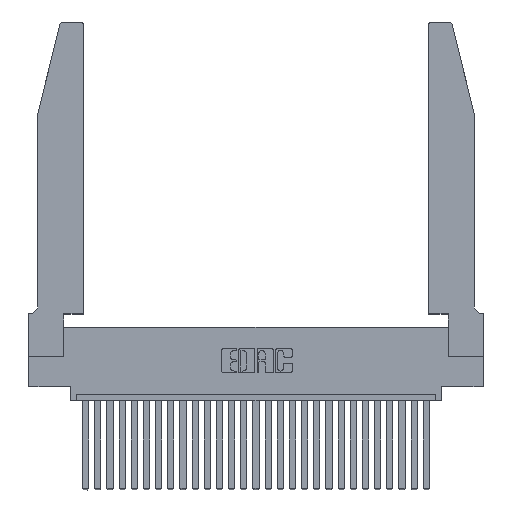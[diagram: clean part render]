
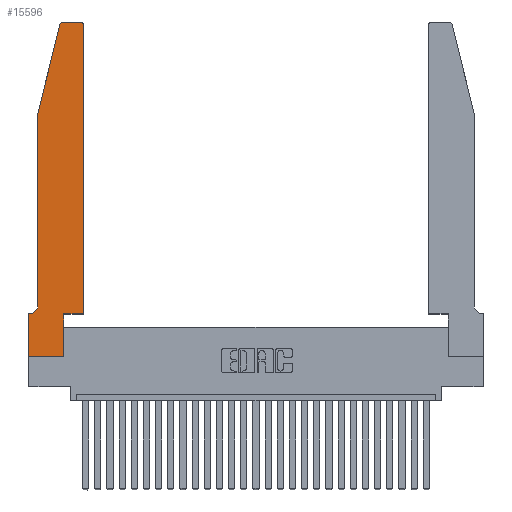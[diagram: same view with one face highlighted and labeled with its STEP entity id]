
A CAD part, top view. The second image highlights one B-rep face of the part: STEP entity #15596.
In plain terms, the highlighted planar face has unit normal (0, 0, 1).
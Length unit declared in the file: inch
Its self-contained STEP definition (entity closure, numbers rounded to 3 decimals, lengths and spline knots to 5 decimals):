
#415 = DIRECTION ( 'NONE',  ( 1., 0., 0. ) ) ;
#1036 = CARTESIAN_POINT ( 'NONE',  ( 0., 0.35, 0.37 ) ) ;
#1130 = LINE ( 'NONE', #27036, #25016 ) ;
#1183 = DIRECTION ( 'NONE',  ( 0., -1., 0. ) ) ;
#1680 = AXIS2_PLACEMENT_3D ( 'NONE', #26564, #13451, #415 ) ;
#1920 = CARTESIAN_POINT ( 'NONE',  ( 0.4505, 0.35, 0.37 ) ) ;
#2234 = VERTEX_POINT ( 'NONE', #7992 ) ;
#2276 = EDGE_CURVE ( 'NONE', #23828, #10349, #15919, .T. ) ;
#2674 = CARTESIAN_POINT ( 'NONE',  ( 0.2865, 0.35, 0.37 ) ) ;
#3351 = CARTESIAN_POINT ( 'NONE',  ( 0.25487, 2.72718, 0.37 ) ) ;
#3857 = VERTEX_POINT ( 'NONE', #1036 ) ;
#3939 = CARTESIAN_POINT ( 'NONE',  ( 0.0755, 2., 0.37 ) ) ;
#4327 = VERTEX_POINT ( 'NONE', #22455 ) ;
#4660 = AXIS2_PLACEMENT_3D ( 'NONE', #6257, #19275, #23594 ) ;
#5125 = CARTESIAN_POINT ( 'NONE',  ( 0.2605, 2.75, 0.37 ) ) ;
#5179 = CARTESIAN_POINT ( 'NONE',  ( 0.2865, 0.35, 0.37 ) ) ;
#5183 = CARTESIAN_POINT ( 'NONE',  ( 0.4505, 2.72, 0.37 ) ) ;
#5343 = VECTOR ( 'NONE', #1183, 39.37008 ) ;
#5871 = ORIENTED_EDGE ( 'NONE', *, *, #2276, .T. ) ;
#6257 = CARTESIAN_POINT ( 'NONE',  ( 0.0055, 0.42, 0.37 ) ) ;
#6505 = CARTESIAN_POINT ( 'NONE',  ( 0.4205, 2.72, 0.37 ) ) ;
#6603 = EDGE_LOOP ( 'NONE', ( #27213, #22534, #7168, #23270, #9719, #13667, #22510, #10000, #21009, #5871, #13877, #24742 ) ) ;
#7168 = ORIENTED_EDGE ( 'NONE', *, *, #11654, .T. ) ;
#7388 = LINE ( 'NONE', #27141, #5343 ) ;
#7731 = DIRECTION ( 'NONE',  ( -0.239, -0.971, 0. ) ) ;
#7992 = CARTESIAN_POINT ( 'NONE',  ( 0., 0., 0.37 ) ) ;
#8528 = VECTOR ( 'NONE', #26946, 39.37008 ) ;
#8648 = EDGE_CURVE ( 'NONE', #10349, #11797, #23971, .T. ) ;
#8759 = CARTESIAN_POINT ( 'NONE',  ( 0.4505, 0.35, 0.37 ) ) ;
#8798 = DIRECTION ( 'NONE',  ( 1., 0., 0. ) ) ;
#8976 = AXIS2_PLACEMENT_3D ( 'NONE', #15329, #25448, #24023 ) ;
#9004 = CARTESIAN_POINT ( 'NONE',  ( 0.0755, 0.42, 0.37 ) ) ;
#9065 = CIRCLE ( 'NONE', #22004, 0.03 ) ;
#9530 = LINE ( 'NONE', #5125, #8528 ) ;
#9719 = ORIENTED_EDGE ( 'NONE', *, *, #20926, .T. ) ;
#9787 = CARTESIAN_POINT ( 'NONE',  ( 0., 0., 0.37 ) ) ;
#10000 = ORIENTED_EDGE ( 'NONE', *, *, #12123, .T. ) ;
#10050 = VECTOR ( 'NONE', #7731, 39.37008 ) ;
#10331 = EDGE_CURVE ( 'NONE', #12961, #4327, #9530, .T. ) ;
#10349 = VERTEX_POINT ( 'NONE', #26844 ) ;
#10372 = DIRECTION ( 'NONE',  ( 1., 0., 0. ) ) ;
#11444 = EDGE_CURVE ( 'NONE', #12896, #23828, #17238, .T. ) ;
#11583 = VERTEX_POINT ( 'NONE', #9004 ) ;
#11654 = EDGE_CURVE ( 'NONE', #22924, #15992, #23799, .T. ) ;
#11797 = VERTEX_POINT ( 'NONE', #5183 ) ;
#12123 = EDGE_CURVE ( 'NONE', #2234, #12896, #21019, .T. ) ;
#12896 = VERTEX_POINT ( 'NONE', #19856 ) ;
#12961 = VERTEX_POINT ( 'NONE', #27208 ) ;
#13053 = EDGE_CURVE ( 'NONE', #4327, #22924, #23366, .T. ) ;
#13451 = DIRECTION ( 'NONE',  ( 0., 0., 1. ) ) ;
#13667 = ORIENTED_EDGE ( 'NONE', *, *, #21769, .T. ) ;
#13877 = ORIENTED_EDGE ( 'NONE', *, *, #8648, .T. ) ;
#14524 = EDGE_CURVE ( 'NONE', #15992, #11583, #7388, .T. ) ;
#14674 = CARTESIAN_POINT ( 'NONE',  ( 0.0055, 0.35, 0.37 ) ) ;
#15329 = CARTESIAN_POINT ( 'NONE',  ( 0., 0.35, 0.37 ) ) ;
#15385 = LINE ( 'NONE', #24969, #17817 ) ;
#15596 = ADVANCED_FACE ( 'NONE', ( #27909 ), #17480, .T. ) ;
#15919 = LINE ( 'NONE', #8759, #25504 ) ;
#15992 = VERTEX_POINT ( 'NONE', #3939 ) ;
#17238 = LINE ( 'NONE', #2674, #23065 ) ;
#17480 = PLANE ( 'NONE',  #8976 ) ;
#17491 = DIRECTION ( 'NONE',  ( 0., 0., 1. ) ) ;
#17817 = VECTOR ( 'NONE', #24889, 39.37008 ) ;
#18172 = VERTEX_POINT ( 'NONE', #14674 ) ;
#19275 = DIRECTION ( 'NONE',  ( 0., 0., -1. ) ) ;
#19856 = CARTESIAN_POINT ( 'NONE',  ( 0.2865, 0., 0.37 ) ) ;
#20667 = CARTESIAN_POINT ( 'NONE',  ( 0.0755, 2., 0.37 ) ) ;
#20926 = EDGE_CURVE ( 'NONE', #11583, #18172, #26381, .T. ) ;
#21009 = ORIENTED_EDGE ( 'NONE', *, *, #11444, .T. ) ;
#21019 = LINE ( 'NONE', #9787, #24769 ) ;
#21495 = EDGE_CURVE ( 'NONE', #3857, #2234, #15385, .T. ) ;
#21769 = EDGE_CURVE ( 'NONE', #18172, #3857, #1130, .T. ) ;
#22004 = AXIS2_PLACEMENT_3D ( 'NONE', #6505, #17491, #8798 ) ;
#22455 = CARTESIAN_POINT ( 'NONE',  ( 0.284, 2.75, 0.37 ) ) ;
#22510 = ORIENTED_EDGE ( 'NONE', *, *, #21495, .T. ) ;
#22534 = ORIENTED_EDGE ( 'NONE', *, *, #13053, .T. ) ;
#22924 = VERTEX_POINT ( 'NONE', #3351 ) ;
#23065 = VECTOR ( 'NONE', #24344, 39.37008 ) ;
#23270 = ORIENTED_EDGE ( 'NONE', *, *, #14524, .T. ) ;
#23366 = CIRCLE ( 'NONE', #1680, 0.03 ) ;
#23594 = DIRECTION ( 'NONE',  ( -1., 0., 0. ) ) ;
#23799 = LINE ( 'NONE', #20667, #10050 ) ;
#23828 = VERTEX_POINT ( 'NONE', #5179 ) ;
#23971 = LINE ( 'NONE', #1920, #27395 ) ;
#24023 = DIRECTION ( 'NONE',  ( 1., 0., 0. ) ) ;
#24058 = DIRECTION ( 'NONE',  ( 1., 0., 0. ) ) ;
#24344 = DIRECTION ( 'NONE',  ( 0., 1., 0. ) ) ;
#24742 = ORIENTED_EDGE ( 'NONE', *, *, #27731, .T. ) ;
#24769 = VECTOR ( 'NONE', #10372, 39.37008 ) ;
#24889 = DIRECTION ( 'NONE',  ( 0., -1., 0. ) ) ;
#24919 = DIRECTION ( 'NONE',  ( -1., 0., 0. ) ) ;
#24969 = CARTESIAN_POINT ( 'NONE',  ( 0., 0., 0.37 ) ) ;
#25016 = VECTOR ( 'NONE', #24919, 39.37008 ) ;
#25448 = DIRECTION ( 'NONE',  ( 0., 0., 1. ) ) ;
#25504 = VECTOR ( 'NONE', #24058, 39.37008 ) ;
#26381 = CIRCLE ( 'NONE', #4660, 0.07 ) ;
#26516 = DIRECTION ( 'NONE',  ( 0., 1., 0. ) ) ;
#26564 = CARTESIAN_POINT ( 'NONE',  ( 0.284, 2.72, 0.37 ) ) ;
#26844 = CARTESIAN_POINT ( 'NONE',  ( 0.4505, 0.35, 0.37 ) ) ;
#26946 = DIRECTION ( 'NONE',  ( -1., 0., 0. ) ) ;
#27036 = CARTESIAN_POINT ( 'NONE',  ( 0.0755, 0.35, 0.37 ) ) ;
#27141 = CARTESIAN_POINT ( 'NONE',  ( 0.0755, 2., 0.37 ) ) ;
#27208 = CARTESIAN_POINT ( 'NONE',  ( 0.4205, 2.75, 0.37 ) ) ;
#27213 = ORIENTED_EDGE ( 'NONE', *, *, #10331, .T. ) ;
#27395 = VECTOR ( 'NONE', #26516, 39.37008 ) ;
#27731 = EDGE_CURVE ( 'NONE', #11797, #12961, #9065, .T. ) ;
#27909 = FACE_OUTER_BOUND ( 'NONE', #6603, .T. ) ;
